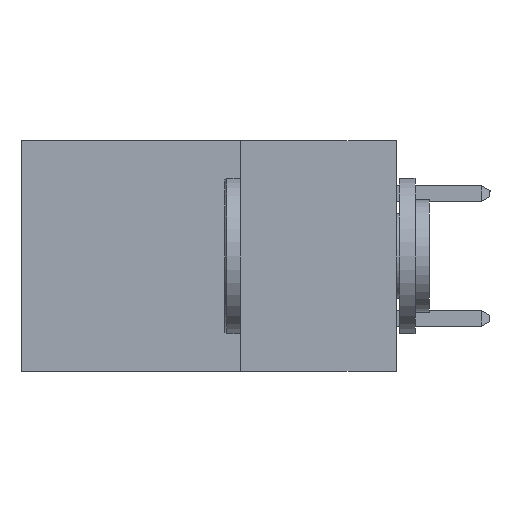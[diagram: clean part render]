
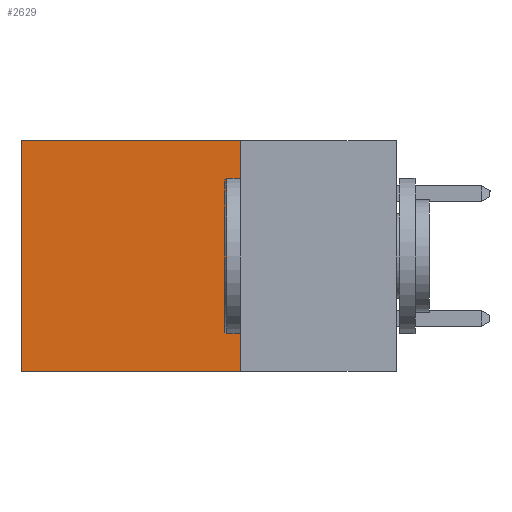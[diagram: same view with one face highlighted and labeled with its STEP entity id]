
A CAD part, left-side view. The second image highlights one B-rep face of the part: STEP entity #2629.
In plain terms, the highlighted planar face has unit normal (-1, 0, 0).
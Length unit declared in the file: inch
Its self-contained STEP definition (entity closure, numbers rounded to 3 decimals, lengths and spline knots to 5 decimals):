
#43 = EDGE_CURVE ( 'NONE', #238, #8522, #12349, .T. ) ;
#238 = VERTEX_POINT ( 'NONE', #2812 ) ;
#1057 = CARTESIAN_POINT ( 'NONE',  ( 0.2615, 0.25, -0.37 ) ) ;
#2112 = EDGE_LOOP ( 'NONE', ( #7658, #3329, #11411, #8607 ) ) ;
#2205 = CARTESIAN_POINT ( 'NONE',  ( 0.2615, 0.25, -0.37 ) ) ;
#2629 = ADVANCED_FACE ( 'NONE', ( #5518 ), #10041, .F. ) ;
#2775 = VECTOR ( 'NONE', #4621, 39.37008 ) ;
#2812 = CARTESIAN_POINT ( 'NONE',  ( 0.2615, 0.25, 0. ) ) ;
#3251 = LINE ( 'NONE', #8630, #13245 ) ;
#3314 = VERTEX_POINT ( 'NONE', #11066 ) ;
#3329 = ORIENTED_EDGE ( 'NONE', *, *, #7621, .F. ) ;
#4148 = CARTESIAN_POINT ( 'NONE',  ( 0.2615, 0.25, -0.37 ) ) ;
#4621 = DIRECTION ( 'NONE',  ( 0., 1., 0. ) ) ;
#4684 = CARTESIAN_POINT ( 'NONE',  ( 0.2615, 0.25, -0.37 ) ) ;
#5518 = FACE_OUTER_BOUND ( 'NONE', #2112, .T. ) ;
#5748 = EDGE_CURVE ( 'NONE', #8522, #3314, #3251, .T. ) ;
#7621 = EDGE_CURVE ( 'NONE', #13021, #3314, #8043, .T. ) ;
#7658 = ORIENTED_EDGE ( 'NONE', *, *, #5748, .T. ) ;
#7807 = CARTESIAN_POINT ( 'NONE',  ( 0.2615, 0.6, 0. ) ) ;
#8043 = LINE ( 'NONE', #4148, #9059 ) ;
#8522 = VERTEX_POINT ( 'NONE', #7807 ) ;
#8567 = DIRECTION ( 'NONE',  ( 0., 1., 0. ) ) ;
#8607 = ORIENTED_EDGE ( 'NONE', *, *, #43, .T. ) ;
#8630 = CARTESIAN_POINT ( 'NONE',  ( 0.2615, 0.6, -0.37 ) ) ;
#9059 = VECTOR ( 'NONE', #8567, 39.37008 ) ;
#9875 = VECTOR ( 'NONE', #12959, 39.37008 ) ;
#10041 = PLANE ( 'NONE',  #11176 ) ;
#10157 = CARTESIAN_POINT ( 'NONE',  ( 0.2615, 0.25, 0. ) ) ;
#10982 = LINE ( 'NONE', #2205, #9875 ) ;
#11066 = CARTESIAN_POINT ( 'NONE',  ( 0.2615, 0.6, -0.37 ) ) ;
#11176 = AXIS2_PLACEMENT_3D ( 'NONE', #1057, #12029, #13113 ) ;
#11411 = ORIENTED_EDGE ( 'NONE', *, *, #13559, .F. ) ;
#12029 = DIRECTION ( 'NONE',  ( 1., 0., 0. ) ) ;
#12349 = LINE ( 'NONE', #10157, #2775 ) ;
#12959 = DIRECTION ( 'NONE',  ( 0., 0., -1. ) ) ;
#13021 = VERTEX_POINT ( 'NONE', #4684 ) ;
#13083 = DIRECTION ( 'NONE',  ( 0., 0., -1. ) ) ;
#13113 = DIRECTION ( 'NONE',  ( 0., 0., -1. ) ) ;
#13245 = VECTOR ( 'NONE', #13083, 39.37008 ) ;
#13559 = EDGE_CURVE ( 'NONE', #238, #13021, #10982, .T. ) ;
